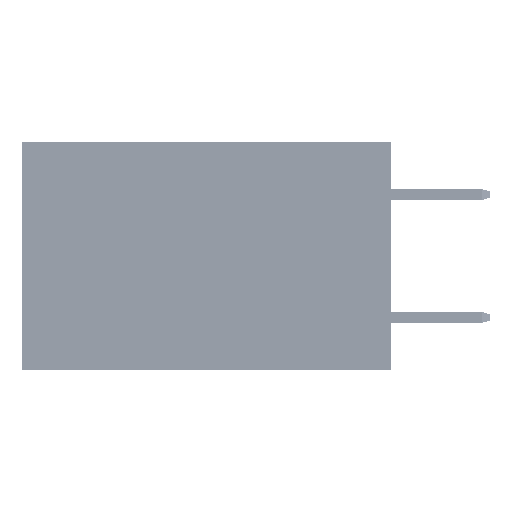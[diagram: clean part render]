
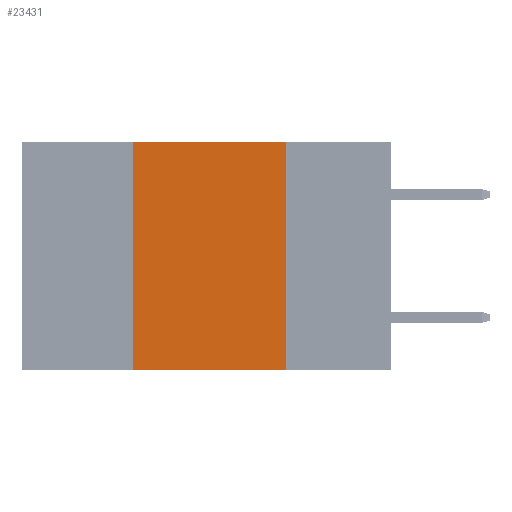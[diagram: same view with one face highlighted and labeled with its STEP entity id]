
A CAD part, left-side view. The second image highlights one B-rep face of the part: STEP entity #23431.
In plain terms, the highlighted planar face has unit normal (-1, 0, 0).
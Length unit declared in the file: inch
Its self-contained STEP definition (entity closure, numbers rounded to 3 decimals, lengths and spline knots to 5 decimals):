
#2019 = VECTOR ( 'NONE', #8189, 39.37008 ) ;
#4191 = DIRECTION ( 'NONE',  ( 0., -1., 0. ) ) ;
#6160 = VERTEX_POINT ( 'NONE', #22241 ) ;
#7394 = CARTESIAN_POINT ( 'NONE',  ( 0., 0.6, 0. ) ) ;
#8189 = DIRECTION ( 'NONE',  ( 0., 0., -1. ) ) ;
#9117 = EDGE_CURVE ( 'NONE', #11554, #34499, #42170, .T. ) ;
#9634 = LINE ( 'NONE', #19883, #2019 ) ;
#10761 = LINE ( 'NONE', #22417, #30474 ) ;
#11011 = EDGE_CURVE ( 'NONE', #6160, #17444, #9634, .T. ) ;
#11041 = CARTESIAN_POINT ( 'NONE',  ( 0., 0.42, 0. ) ) ;
#11131 = DIRECTION ( 'NONE',  ( 0., -1., 0. ) ) ;
#11554 = VERTEX_POINT ( 'NONE', #29942 ) ;
#13169 = CARTESIAN_POINT ( 'NONE',  ( 0., 0.42, 0. ) ) ;
#16099 = VECTOR ( 'NONE', #16897, 39.37008 ) ;
#16897 = DIRECTION ( 'NONE',  ( 0., 0., 1. ) ) ;
#17444 = VERTEX_POINT ( 'NONE', #18021 ) ;
#18021 = CARTESIAN_POINT ( 'NONE',  ( 0., 0.17, -0.37 ) ) ;
#19883 = CARTESIAN_POINT ( 'NONE',  ( 0., 0.17, 0. ) ) ;
#22241 = CARTESIAN_POINT ( 'NONE',  ( 0., 0.17, 0. ) ) ;
#22417 = CARTESIAN_POINT ( 'NONE',  ( 0., 0.6, -0.37 ) ) ;
#23084 = ORIENTED_EDGE ( 'NONE', *, *, #9117, .F. ) ;
#23431 = ADVANCED_FACE ( 'NONE', ( #27863 ), #39460, .F. ) ;
#26332 = EDGE_CURVE ( 'NONE', #11554, #17444, #10761, .T. ) ;
#27863 = FACE_OUTER_BOUND ( 'NONE', #28870, .T. ) ;
#28870 = EDGE_LOOP ( 'NONE', ( #44682, #39065, #23084, #45214 ) ) ;
#28974 = VECTOR ( 'NONE', #11131, 39.37008 ) ;
#29942 = CARTESIAN_POINT ( 'NONE',  ( 0., 0.42, -0.37 ) ) ;
#30474 = VECTOR ( 'NONE', #4191, 39.37008 ) ;
#31286 = LINE ( 'NONE', #7394, #28974 ) ;
#34499 = VERTEX_POINT ( 'NONE', #11041 ) ;
#38123 = AXIS2_PLACEMENT_3D ( 'NONE', #47357, #43621, #43315 ) ;
#39065 = ORIENTED_EDGE ( 'NONE', *, *, #45541, .F. ) ;
#39460 = PLANE ( 'NONE',  #38123 ) ;
#42170 = LINE ( 'NONE', #13169, #16099 ) ;
#43315 = DIRECTION ( 'NONE',  ( 0., 0., -1. ) ) ;
#43621 = DIRECTION ( 'NONE',  ( 1., 0., 0. ) ) ;
#44682 = ORIENTED_EDGE ( 'NONE', *, *, #11011, .F. ) ;
#45214 = ORIENTED_EDGE ( 'NONE', *, *, #26332, .T. ) ;
#45541 = EDGE_CURVE ( 'NONE', #34499, #6160, #31286, .T. ) ;
#47357 = CARTESIAN_POINT ( 'NONE',  ( 0., 0.6, 0. ) ) ;
